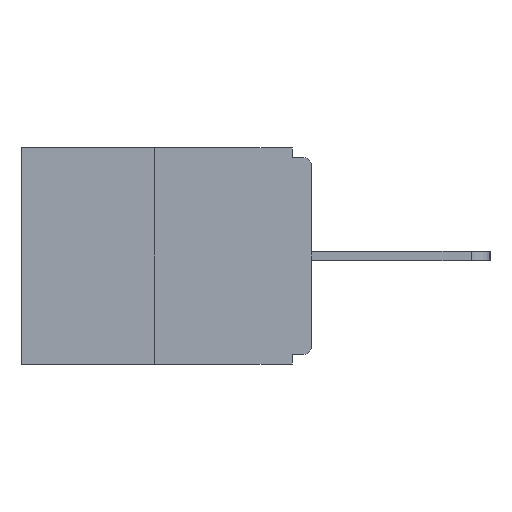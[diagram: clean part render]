
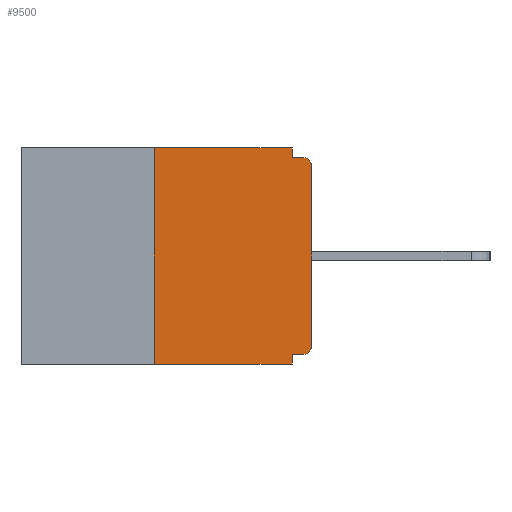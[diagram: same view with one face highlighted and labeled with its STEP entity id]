
A CAD part, left-side view. The second image highlights one B-rep face of the part: STEP entity #9500.
In plain terms, the highlighted planar face has unit normal (-1, 0, 0).
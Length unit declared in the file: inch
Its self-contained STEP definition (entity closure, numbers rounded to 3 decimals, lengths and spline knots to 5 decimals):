
#63 = ORIENTED_EDGE ( 'NONE', *, *, #15395, .T. ) ;
#485 = VERTEX_POINT ( 'NONE', #18187 ) ;
#497 = CARTESIAN_POINT ( 'NONE',  ( 0., 0., -0.03 ) ) ;
#537 = DIRECTION ( 'NONE',  ( -1., 0., 0. ) ) ;
#567 = CARTESIAN_POINT ( 'NONE',  ( 0., 0., 0. ) ) ;
#709 = CARTESIAN_POINT ( 'NONE',  ( 0., 0.46, 0. ) ) ;
#843 = VERTEX_POINT ( 'NONE', #12855 ) ;
#1165 = LINE ( 'NONE', #19559, #12690 ) ;
#1414 = CARTESIAN_POINT ( 'NONE',  ( 0., 0.25, -0.343 ) ) ;
#1507 = ORIENTED_EDGE ( 'NONE', *, *, #14876, .F. ) ;
#1914 = EDGE_CURVE ( 'NONE', #2899, #18934, #3456, .T. ) ;
#2040 = CARTESIAN_POINT ( 'NONE',  ( 0., 0.015, -0.313 ) ) ;
#2195 = CARTESIAN_POINT ( 'NONE',  ( 0., 0.031, -0.343 ) ) ;
#2217 = CARTESIAN_POINT ( 'NONE',  ( 0., 0., -0.313 ) ) ;
#2462 = ORIENTED_EDGE ( 'NONE', *, *, #1914, .T. ) ;
#2899 = VERTEX_POINT ( 'NONE', #2217 ) ;
#3326 = AXIS2_PLACEMENT_3D ( 'NONE', #2040, #537, #6577 ) ;
#3359 = EDGE_CURVE ( 'NONE', #843, #10926, #14290, .T. ) ;
#3396 = VERTEX_POINT ( 'NONE', #4962 ) ;
#3456 = LINE ( 'NONE', #567, #12870 ) ;
#3985 = CARTESIAN_POINT ( 'NONE',  ( 0., 0.46, 0. ) ) ;
#4051 = DIRECTION ( 'NONE',  ( 0., 0., -1. ) ) ;
#4256 = CARTESIAN_POINT ( 'NONE',  ( 0., 0.015, -0.03 ) ) ;
#4520 = CIRCLE ( 'NONE', #17575, 0.015 ) ;
#4617 = VERTEX_POINT ( 'NONE', #1414 ) ;
#4781 = CARTESIAN_POINT ( 'NONE',  ( 0., 0.015, -0.015 ) ) ;
#4962 = CARTESIAN_POINT ( 'NONE',  ( 0., 0.015, -0.328 ) ) ;
#5091 = LINE ( 'NONE', #11159, #10541 ) ;
#5346 = VECTOR ( 'NONE', #18596, 39.37008 ) ;
#5517 = CARTESIAN_POINT ( 'NONE',  ( 0., 0.031, 0. ) ) ;
#5583 = DIRECTION ( 'NONE',  ( 1., 0., 0. ) ) ;
#5664 = AXIS2_PLACEMENT_3D ( 'NONE', #3985, #5583, #6770 ) ;
#5890 = EDGE_CURVE ( 'NONE', #3396, #843, #19231, .T. ) ;
#6494 = VERTEX_POINT ( 'NONE', #4781 ) ;
#6577 = DIRECTION ( 'NONE',  ( 0., 0., -1. ) ) ;
#6770 = DIRECTION ( 'NONE',  ( 0., 0., -1. ) ) ;
#7026 = DIRECTION ( 'NONE',  ( -1., 0., 0. ) ) ;
#7290 = DIRECTION ( 'NONE',  ( 0., 0., -1. ) ) ;
#7457 = CARTESIAN_POINT ( 'NONE',  ( 0., 0.031, -0.343 ) ) ;
#7744 = CIRCLE ( 'NONE', #3326, 0.015 ) ;
#8074 = EDGE_CURVE ( 'NONE', #12677, #13906, #17413, .T. ) ;
#9219 = CARTESIAN_POINT ( 'NONE',  ( 0., 0.25, 0. ) ) ;
#9500 = ADVANCED_FACE ( 'NONE', ( #12828 ), #16236, .F. ) ;
#9982 = LINE ( 'NONE', #11672, #14937 ) ;
#10274 = EDGE_LOOP ( 'NONE', ( #13934, #10980, #19029, #16037, #13409, #12473, #2462, #63, #1507, #14721 ) ) ;
#10281 = DIRECTION ( 'NONE',  ( 0., -1., 0. ) ) ;
#10362 = EDGE_CURVE ( 'NONE', #13906, #485, #19441, .T. ) ;
#10541 = VECTOR ( 'NONE', #17238, 39.37008 ) ;
#10926 = VERTEX_POINT ( 'NONE', #7457 ) ;
#10980 = ORIENTED_EDGE ( 'NONE', *, *, #12630, .F. ) ;
#11159 = CARTESIAN_POINT ( 'NONE',  ( 0., 0., -0.015 ) ) ;
#11231 = DIRECTION ( 'NONE',  ( 0., -1., 0. ) ) ;
#11399 = VECTOR ( 'NONE', #7290, 39.37008 ) ;
#11628 = VECTOR ( 'NONE', #14746, 39.37008 ) ;
#11672 = CARTESIAN_POINT ( 'NONE',  ( 0., 0.46, -0.343 ) ) ;
#11992 = DIRECTION ( 'NONE',  ( 0., 0., 1. ) ) ;
#12318 = CARTESIAN_POINT ( 'NONE',  ( 0., 0.031, 0. ) ) ;
#12473 = ORIENTED_EDGE ( 'NONE', *, *, #16930, .T. ) ;
#12630 = EDGE_CURVE ( 'NONE', #4617, #12677, #1165, .T. ) ;
#12677 = VERTEX_POINT ( 'NONE', #9219 ) ;
#12690 = VECTOR ( 'NONE', #11992, 39.37008 ) ;
#12828 = FACE_OUTER_BOUND ( 'NONE', #10274, .T. ) ;
#12855 = CARTESIAN_POINT ( 'NONE',  ( 0., 0.031, -0.328 ) ) ;
#12870 = VECTOR ( 'NONE', #13870, 39.37008 ) ;
#13032 = EDGE_CURVE ( 'NONE', #4617, #10926, #9982, .T. ) ;
#13228 = VECTOR ( 'NONE', #11231, 39.37008 ) ;
#13409 = ORIENTED_EDGE ( 'NONE', *, *, #5890, .F. ) ;
#13870 = DIRECTION ( 'NONE',  ( 0., 0., 1. ) ) ;
#13906 = VERTEX_POINT ( 'NONE', #12318 ) ;
#13934 = ORIENTED_EDGE ( 'NONE', *, *, #8074, .F. ) ;
#14290 = LINE ( 'NONE', #2195, #5346 ) ;
#14721 = ORIENTED_EDGE ( 'NONE', *, *, #10362, .F. ) ;
#14746 = DIRECTION ( 'NONE',  ( 0., 1., 0. ) ) ;
#14876 = EDGE_CURVE ( 'NONE', #485, #6494, #5091, .T. ) ;
#14937 = VECTOR ( 'NONE', #10281, 39.37008 ) ;
#15395 = EDGE_CURVE ( 'NONE', #18934, #6494, #4520, .T. ) ;
#16037 = ORIENTED_EDGE ( 'NONE', *, *, #3359, .F. ) ;
#16236 = PLANE ( 'NONE',  #5664 ) ;
#16930 = EDGE_CURVE ( 'NONE', #3396, #2899, #7744, .T. ) ;
#17238 = DIRECTION ( 'NONE',  ( 0., -1., 0. ) ) ;
#17413 = LINE ( 'NONE', #709, #13228 ) ;
#17564 = CARTESIAN_POINT ( 'NONE',  ( 0., 0., -0.328 ) ) ;
#17575 = AXIS2_PLACEMENT_3D ( 'NONE', #4256, #7026, #4051 ) ;
#18187 = CARTESIAN_POINT ( 'NONE',  ( 0., 0.031, -0.015 ) ) ;
#18596 = DIRECTION ( 'NONE',  ( 0., 0., -1. ) ) ;
#18934 = VERTEX_POINT ( 'NONE', #497 ) ;
#19029 = ORIENTED_EDGE ( 'NONE', *, *, #13032, .T. ) ;
#19231 = LINE ( 'NONE', #17564, #11628 ) ;
#19441 = LINE ( 'NONE', #5517, #11399 ) ;
#19559 = CARTESIAN_POINT ( 'NONE',  ( 0., 0.25, 0. ) ) ;
